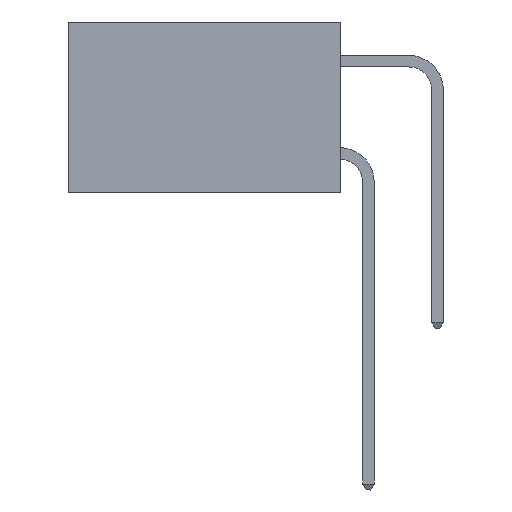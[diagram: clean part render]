
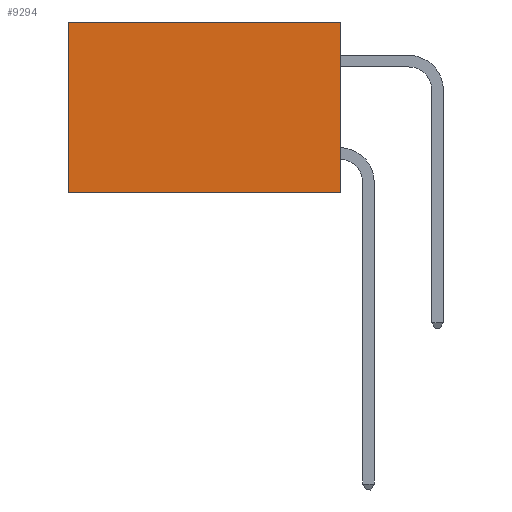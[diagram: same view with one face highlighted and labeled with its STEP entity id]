
A CAD part, left-side view. The second image highlights one B-rep face of the part: STEP entity #9294.
In plain terms, the highlighted planar face has unit normal (-1, 0, 0).
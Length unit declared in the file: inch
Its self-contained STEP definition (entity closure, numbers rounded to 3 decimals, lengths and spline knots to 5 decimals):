
#224 = CARTESIAN_POINT ( 'NONE',  ( 0.277, 0.59, -0.37 ) ) ;
#1122 = LINE ( 'NONE', #9452, #12014 ) ;
#1174 = LINE ( 'NONE', #6451, #8747 ) ;
#2487 = EDGE_CURVE ( 'NONE', #14386, #16963, #1174, .T. ) ;
#2801 = ORIENTED_EDGE ( 'NONE', *, *, #3381, .T. ) ;
#3381 = EDGE_CURVE ( 'NONE', #5472, #5629, #4735, .T. ) ;
#4330 = CARTESIAN_POINT ( 'NONE',  ( 0.277, 0.59, -0.37 ) ) ;
#4735 = LINE ( 'NONE', #11786, #7607 ) ;
#4785 = ORIENTED_EDGE ( 'NONE', *, *, #10078, .F. ) ;
#4808 = CARTESIAN_POINT ( 'NONE',  ( 0.277, 0., -0.37 ) ) ;
#5287 = CARTESIAN_POINT ( 'NONE',  ( 0.277, 0.59, 0. ) ) ;
#5387 = DIRECTION ( 'NONE',  ( 0., 1., 0. ) ) ;
#5472 = VERTEX_POINT ( 'NONE', #13443 ) ;
#5629 = VERTEX_POINT ( 'NONE', #5287 ) ;
#6451 = CARTESIAN_POINT ( 'NONE',  ( 0.277, 0., -0.37 ) ) ;
#7607 = VECTOR ( 'NONE', #5387, 39.37008 ) ;
#7649 = DIRECTION ( 'NONE',  ( 0., 0., -1. ) ) ;
#7696 = DIRECTION ( 'NONE',  ( 0., 1., 0. ) ) ;
#8741 = ORIENTED_EDGE ( 'NONE', *, *, #9094, .T. ) ;
#8747 = VECTOR ( 'NONE', #7696, 39.37008 ) ;
#9094 = EDGE_CURVE ( 'NONE', #5629, #16963, #16354, .T. ) ;
#9294 = ADVANCED_FACE ( 'NONE', ( #13734 ), #14683, .F. ) ;
#9452 = CARTESIAN_POINT ( 'NONE',  ( 0.277, 0., -0.37 ) ) ;
#10078 = EDGE_CURVE ( 'NONE', #5472, #14386, #1122, .T. ) ;
#10108 = DIRECTION ( 'NONE',  ( 0., 0., -1. ) ) ;
#10373 = ORIENTED_EDGE ( 'NONE', *, *, #2487, .F. ) ;
#11786 = CARTESIAN_POINT ( 'NONE',  ( 0.277, 0., 0. ) ) ;
#12014 = VECTOR ( 'NONE', #17770, 39.37008 ) ;
#12249 = AXIS2_PLACEMENT_3D ( 'NONE', #4808, #16073, #7649 ) ;
#13108 = VECTOR ( 'NONE', #10108, 39.37008 ) ;
#13443 = CARTESIAN_POINT ( 'NONE',  ( 0.277, 0., 0. ) ) ;
#13734 = FACE_OUTER_BOUND ( 'NONE', #17058, .T. ) ;
#14386 = VERTEX_POINT ( 'NONE', #14848 ) ;
#14683 = PLANE ( 'NONE',  #12249 ) ;
#14848 = CARTESIAN_POINT ( 'NONE',  ( 0.277, 0., -0.37 ) ) ;
#16073 = DIRECTION ( 'NONE',  ( 1., 0., 0. ) ) ;
#16354 = LINE ( 'NONE', #224, #13108 ) ;
#16963 = VERTEX_POINT ( 'NONE', #4330 ) ;
#17058 = EDGE_LOOP ( 'NONE', ( #8741, #10373, #4785, #2801 ) ) ;
#17770 = DIRECTION ( 'NONE',  ( 0., 0., -1. ) ) ;
